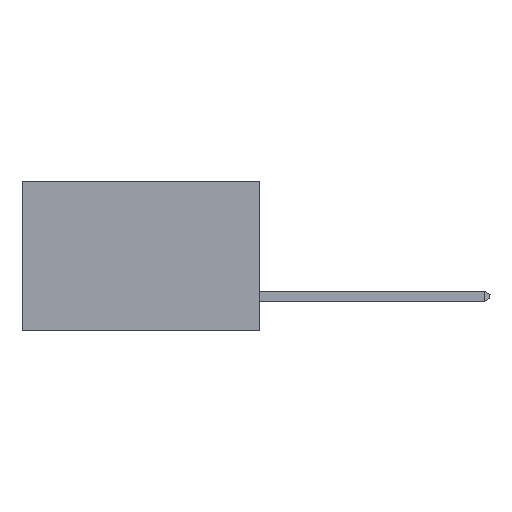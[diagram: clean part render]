
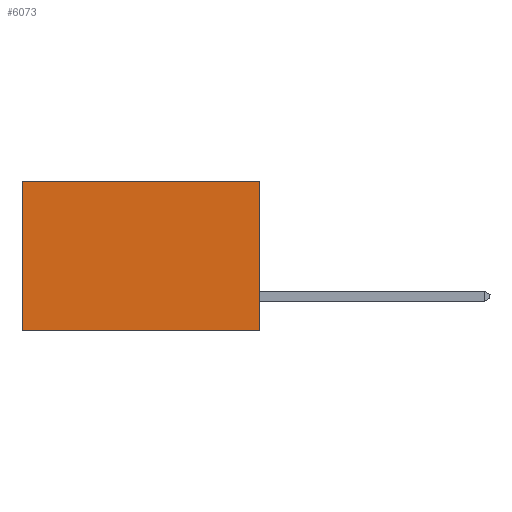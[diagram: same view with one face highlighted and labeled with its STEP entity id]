
A CAD part, left-side view. The second image highlights one B-rep face of the part: STEP entity #6073.
In plain terms, the highlighted planar face has unit normal (-1, 0, 0).
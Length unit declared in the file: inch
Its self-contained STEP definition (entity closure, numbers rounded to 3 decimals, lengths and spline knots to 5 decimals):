
#66 = DIRECTION ( 'NONE',  ( 0., 1., 0. ) ) ;
#198 = VERTEX_POINT ( 'NONE', #7620 ) ;
#967 = ORIENTED_EDGE ( 'NONE', *, *, #9342, .T. ) ;
#1422 = DIRECTION ( 'NONE',  ( 0., 0., -1. ) ) ;
#2018 = CARTESIAN_POINT ( 'NONE',  ( 0.277, 0., -0.37 ) ) ;
#2793 = VECTOR ( 'NONE', #66, 39.37008 ) ;
#3120 = EDGE_CURVE ( 'NONE', #198, #3865, #7739, .T. ) ;
#3766 = CARTESIAN_POINT ( 'NONE',  ( 0.277, 0.59, 0. ) ) ;
#3865 = VERTEX_POINT ( 'NONE', #3766 ) ;
#3969 = LINE ( 'NONE', #7113, #10833 ) ;
#4556 = VECTOR ( 'NONE', #1422, 39.37008 ) ;
#4565 = FACE_OUTER_BOUND ( 'NONE', #5962, .T. ) ;
#5494 = AXIS2_PLACEMENT_3D ( 'NONE', #5782, #6979, #6959 ) ;
#5669 = EDGE_CURVE ( 'NONE', #7850, #10169, #3969, .T. ) ;
#5691 = ORIENTED_EDGE ( 'NONE', *, *, #5669, .F. ) ;
#5782 = CARTESIAN_POINT ( 'NONE',  ( 0.277, 0., -0.37 ) ) ;
#5949 = ORIENTED_EDGE ( 'NONE', *, *, #3120, .T. ) ;
#5962 = EDGE_LOOP ( 'NONE', ( #967, #5691, #8658, #5949 ) ) ;
#6073 = ADVANCED_FACE ( 'NONE', ( #4565 ), #6763, .F. ) ;
#6165 = VECTOR ( 'NONE', #8054, 39.37008 ) ;
#6763 = PLANE ( 'NONE',  #5494 ) ;
#6959 = DIRECTION ( 'NONE',  ( 0., 0., -1. ) ) ;
#6971 = CARTESIAN_POINT ( 'NONE',  ( 0.277, 0., -0.37 ) ) ;
#6979 = DIRECTION ( 'NONE',  ( 1., 0., 0. ) ) ;
#7113 = CARTESIAN_POINT ( 'NONE',  ( 0.277, 0., -0.37 ) ) ;
#7144 = CARTESIAN_POINT ( 'NONE',  ( 0.277, 0.59, -0.37 ) ) ;
#7620 = CARTESIAN_POINT ( 'NONE',  ( 0.277, 0., 0. ) ) ;
#7721 = DIRECTION ( 'NONE',  ( 0., 1., 0. ) ) ;
#7739 = LINE ( 'NONE', #10108, #2793 ) ;
#7850 = VERTEX_POINT ( 'NONE', #2018 ) ;
#8054 = DIRECTION ( 'NONE',  ( 0., 0., -1. ) ) ;
#8658 = ORIENTED_EDGE ( 'NONE', *, *, #10274, .F. ) ;
#9342 = EDGE_CURVE ( 'NONE', #3865, #10169, #10823, .T. ) ;
#10108 = CARTESIAN_POINT ( 'NONE',  ( 0.277, 0., 0. ) ) ;
#10169 = VERTEX_POINT ( 'NONE', #11076 ) ;
#10274 = EDGE_CURVE ( 'NONE', #198, #7850, #11334, .T. ) ;
#10823 = LINE ( 'NONE', #7144, #6165 ) ;
#10833 = VECTOR ( 'NONE', #7721, 39.37008 ) ;
#11076 = CARTESIAN_POINT ( 'NONE',  ( 0.277, 0.59, -0.37 ) ) ;
#11334 = LINE ( 'NONE', #6971, #4556 ) ;
